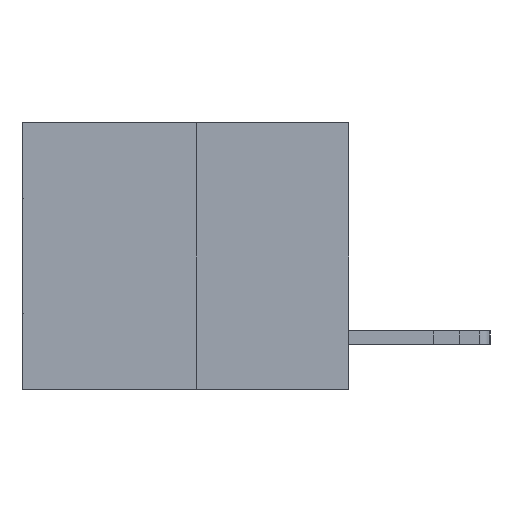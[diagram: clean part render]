
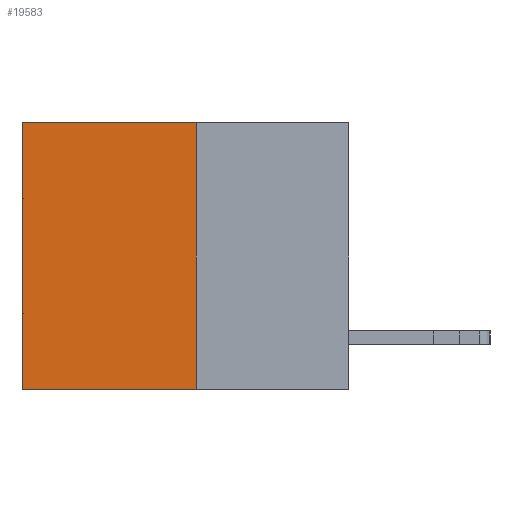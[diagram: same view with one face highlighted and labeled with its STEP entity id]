
A CAD part, left-side view. The second image highlights one B-rep face of the part: STEP entity #19583.
In plain terms, the highlighted planar face has unit normal (-1, 0, 0).
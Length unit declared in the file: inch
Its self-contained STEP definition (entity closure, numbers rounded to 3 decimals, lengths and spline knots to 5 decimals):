
#727 = FACE_OUTER_BOUND ( 'NONE', #5185, .T. ) ;
#1078 = CARTESIAN_POINT ( 'NONE',  ( 0.3165, 0.28, 0. ) ) ;
#1546 = DIRECTION ( 'NONE',  ( 0., 0., -1. ) ) ;
#2835 = EDGE_CURVE ( 'NONE', #12387, #18708, #11191, .T. ) ;
#4775 = DIRECTION ( 'NONE',  ( 0., 1., 0. ) ) ;
#5185 = EDGE_LOOP ( 'NONE', ( #26844, #8755, #15268, #19768 ) ) ;
#6694 = DIRECTION ( 'NONE',  ( 0., 0., -1. ) ) ;
#6865 = DIRECTION ( 'NONE',  ( 0., 1., 0. ) ) ;
#8755 = ORIENTED_EDGE ( 'NONE', *, *, #13828, .F. ) ;
#8924 = VECTOR ( 'NONE', #22145, 39.37008 ) ;
#11191 = LINE ( 'NONE', #20438, #18439 ) ;
#12165 = EDGE_CURVE ( 'NONE', #18708, #15271, #23574, .T. ) ;
#12387 = VERTEX_POINT ( 'NONE', #1078 ) ;
#12987 = CARTESIAN_POINT ( 'NONE',  ( 0.3165, 0.6, -0.49 ) ) ;
#13828 = EDGE_CURVE ( 'NONE', #15991, #15271, #20977, .T. ) ;
#15268 = ORIENTED_EDGE ( 'NONE', *, *, #26347, .F. ) ;
#15271 = VERTEX_POINT ( 'NONE', #12987 ) ;
#15991 = VERTEX_POINT ( 'NONE', #17535 ) ;
#16592 = CARTESIAN_POINT ( 'NONE',  ( 0.3165, 0.6, 0. ) ) ;
#17535 = CARTESIAN_POINT ( 'NONE',  ( 0.3165, 0.28, -0.49 ) ) ;
#18439 = VECTOR ( 'NONE', #6865, 39.37008 ) ;
#18656 = CARTESIAN_POINT ( 'NONE',  ( 0.3165, 0.28, -0.49 ) ) ;
#18708 = VERTEX_POINT ( 'NONE', #16592 ) ;
#18813 = VECTOR ( 'NONE', #4775, 39.37008 ) ;
#19583 = ADVANCED_FACE ( 'NONE', ( #727 ), #23168, .F. ) ;
#19768 = ORIENTED_EDGE ( 'NONE', *, *, #2835, .T. ) ;
#20438 = CARTESIAN_POINT ( 'NONE',  ( 0.3165, 0.28, 0. ) ) ;
#20565 = DIRECTION ( 'NONE',  ( 1., 0., 0. ) ) ;
#20977 = LINE ( 'NONE', #18656, #18813 ) ;
#22145 = DIRECTION ( 'NONE',  ( 0., 0., -1. ) ) ;
#23168 = PLANE ( 'NONE',  #26771 ) ;
#23574 = LINE ( 'NONE', #26766, #24664 ) ;
#24664 = VECTOR ( 'NONE', #1546, 39.37008 ) ;
#26347 = EDGE_CURVE ( 'NONE', #12387, #15991, #26947, .T. ) ;
#26766 = CARTESIAN_POINT ( 'NONE',  ( 0.3165, 0.6, -0.49 ) ) ;
#26771 = AXIS2_PLACEMENT_3D ( 'NONE', #27677, #20565, #6694 ) ;
#26844 = ORIENTED_EDGE ( 'NONE', *, *, #12165, .T. ) ;
#26947 = LINE ( 'NONE', #28804, #8924 ) ;
#27677 = CARTESIAN_POINT ( 'NONE',  ( 0.3165, 0.28, -0.49 ) ) ;
#28804 = CARTESIAN_POINT ( 'NONE',  ( 0.3165, 0.28, -0.49 ) ) ;
